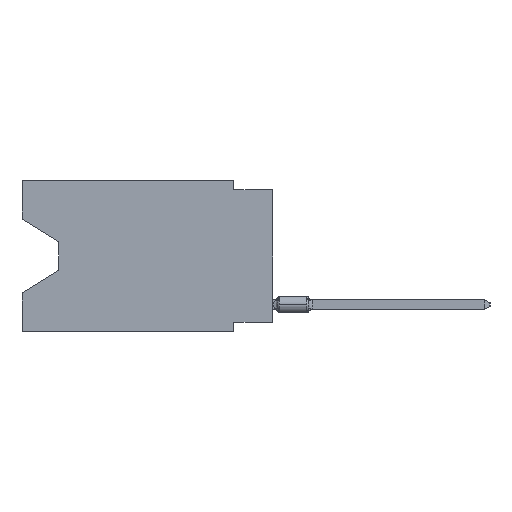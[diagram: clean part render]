
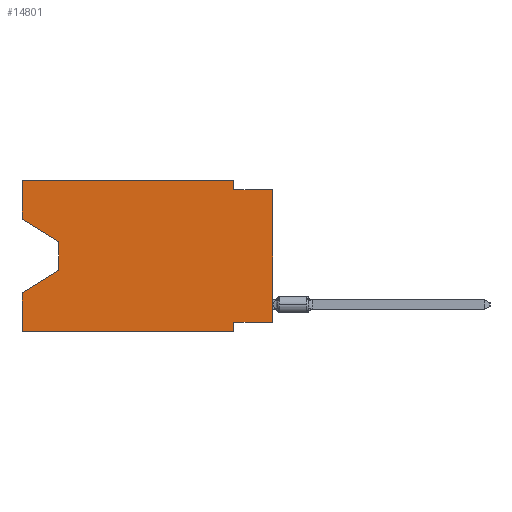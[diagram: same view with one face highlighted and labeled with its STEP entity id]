
A CAD part, left-side view. The second image highlights one B-rep face of the part: STEP entity #14801.
In plain terms, the highlighted planar face has unit normal (-1, 0, 0).
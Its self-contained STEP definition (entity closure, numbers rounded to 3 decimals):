
#1022 = EDGE_CURVE ( 'NONE', #17981, #5788, #20711, .T. ) ;
#1270 = VECTOR ( 'NONE', #9001, 1000. ) ;
#1369 = EDGE_CURVE ( 'NONE', #8016, #17981, #29683, .T. ) ;
#1737 = LINE ( 'NONE', #30207, #1270 ) ;
#1880 = VERTEX_POINT ( 'NONE', #11220 ) ;
#2065 = DIRECTION ( 'NONE',  ( 0., 0., -1. ) ) ;
#2238 = CARTESIAN_POINT ( 'NONE',  ( 0., 0., 0. ) ) ;
#2317 = CARTESIAN_POINT ( 'NONE',  ( 0., 0., -9.271 ) ) ;
#2870 = ORIENTED_EDGE ( 'NONE', *, *, #5244, .F. ) ;
#3889 = VERTEX_POINT ( 'NONE', #9206 ) ;
#4088 = VECTOR ( 'NONE', #12786, 1000. ) ;
#4113 = VECTOR ( 'NONE', #10424, 1000. ) ;
#4931 = LINE ( 'NONE', #23221, #11529 ) ;
#4990 = EDGE_CURVE ( 'NONE', #3889, #19101, #4931, .T. ) ;
#5244 = EDGE_CURVE ( 'NONE', #27262, #8016, #30579, .T. ) ;
#5245 = CARTESIAN_POINT ( 'NONE',  ( 0., 0., -0.635 ) ) ;
#5788 = VERTEX_POINT ( 'NONE', #13596 ) ;
#8016 = VERTEX_POINT ( 'NONE', #12560 ) ;
#8022 = CARTESIAN_POINT ( 'NONE',  ( 0., 16.383, 0. ) ) ;
#8332 = DIRECTION ( 'NONE',  ( 0., -1., 0. ) ) ;
#8886 = ORIENTED_EDGE ( 'NONE', *, *, #13821, .F. ) ;
#9001 = DIRECTION ( 'NONE',  ( 0., 0.855, -0.519 ) ) ;
#9114 = CARTESIAN_POINT ( 'NONE',  ( 0., 2.54, -9.906 ) ) ;
#9206 = CARTESIAN_POINT ( 'NONE',  ( 0., 13.97, -4.013 ) ) ;
#9372 = DIRECTION ( 'NONE',  ( 0., 0., 1. ) ) ;
#9789 = EDGE_CURVE ( 'NONE', #27262, #3889, #12582, .T. ) ;
#10093 = EDGE_CURVE ( 'NONE', #19101, #22108, #1737, .T. ) ;
#10105 = CARTESIAN_POINT ( 'NONE',  ( 0., 16.383, -2.546 ) ) ;
#10164 = LINE ( 'NONE', #24702, #4088 ) ;
#10324 = CARTESIAN_POINT ( 'NONE',  ( 0., 13.97, -5.893 ) ) ;
#10424 = DIRECTION ( 'NONE',  ( 0., 0., 1. ) ) ;
#10769 = VERTEX_POINT ( 'NONE', #9114 ) ;
#11010 = CARTESIAN_POINT ( 'NONE',  ( 0., 2.54, -9.271 ) ) ;
#11053 = FACE_OUTER_BOUND ( 'NONE', #19611, .T. ) ;
#11220 = CARTESIAN_POINT ( 'NONE',  ( 0., 0., -0.635 ) ) ;
#11428 = CARTESIAN_POINT ( 'NONE',  ( 0., 16.383, -9.906 ) ) ;
#11510 = ORIENTED_EDGE ( 'NONE', *, *, #22002, .T. ) ;
#11529 = VECTOR ( 'NONE', #14370, 1000. ) ;
#11697 = CARTESIAN_POINT ( 'NONE',  ( 0., 16.383, 0. ) ) ;
#12560 = CARTESIAN_POINT ( 'NONE',  ( 0., 16.383, 0. ) ) ;
#12582 = LINE ( 'NONE', #10105, #28963 ) ;
#12786 = DIRECTION ( 'NONE',  ( 0., 0., -1. ) ) ;
#13006 = ORIENTED_EDGE ( 'NONE', *, *, #17110, .F. ) ;
#13370 = PLANE ( 'NONE',  #16900 ) ;
#13426 = CARTESIAN_POINT ( 'NONE',  ( 0., 2.54, 0. ) ) ;
#13473 = VECTOR ( 'NONE', #23375, 1000. ) ;
#13487 = ORIENTED_EDGE ( 'NONE', *, *, #1369, .F. ) ;
#13596 = CARTESIAN_POINT ( 'NONE',  ( 0., 2.54, -0.635 ) ) ;
#13754 = CARTESIAN_POINT ( 'NONE',  ( 0., 16.383, -9.906 ) ) ;
#13759 = LINE ( 'NONE', #11428, #17284 ) ;
#13821 = EDGE_CURVE ( 'NONE', #24802, #10769, #10164, .T. ) ;
#14370 = DIRECTION ( 'NONE',  ( 0., 0., -1. ) ) ;
#14801 = ADVANCED_FACE ( 'NONE', ( #11053 ), #13370, .F. ) ;
#14821 = CARTESIAN_POINT ( 'NONE',  ( 0., 16.383, -7.36 ) ) ;
#14868 = VECTOR ( 'NONE', #30140, 1000. ) ;
#14977 = DIRECTION ( 'NONE',  ( 0., -1., 0. ) ) ;
#15236 = CARTESIAN_POINT ( 'NONE',  ( 0., 16.383, 0. ) ) ;
#15493 = VECTOR ( 'NONE', #9372, 1000. ) ;
#16236 = DIRECTION ( 'NONE',  ( 0., -1., 0. ) ) ;
#16244 = CARTESIAN_POINT ( 'NONE',  ( 0., 2.54, 0. ) ) ;
#16626 = DIRECTION ( 'NONE',  ( 0., 0., 1. ) ) ;
#16900 = AXIS2_PLACEMENT_3D ( 'NONE', #20345, #18012, #2065 ) ;
#17066 = VECTOR ( 'NONE', #16626, 1000. ) ;
#17110 = EDGE_CURVE ( 'NONE', #5788, #1880, #26584, .T. ) ;
#17284 = VECTOR ( 'NONE', #16236, 1000. ) ;
#17375 = ORIENTED_EDGE ( 'NONE', *, *, #4990, .T. ) ;
#17699 = LINE ( 'NONE', #15236, #4113 ) ;
#17981 = VERTEX_POINT ( 'NONE', #16244 ) ;
#18012 = DIRECTION ( 'NONE',  ( 1., 0., 0. ) ) ;
#18861 = ORIENTED_EDGE ( 'NONE', *, *, #10093, .T. ) ;
#19101 = VERTEX_POINT ( 'NONE', #10324 ) ;
#19524 = VECTOR ( 'NONE', #14977, 1000. ) ;
#19566 = DIRECTION ( 'NONE',  ( 0., -0.855, -0.519 ) ) ;
#19611 = EDGE_LOOP ( 'NONE', ( #29803, #17375, #18861, #23090, #11510, #8886, #23498, #21616, #13006, #20417, #13487, #2870 ) ) ;
#19881 = CARTESIAN_POINT ( 'NONE',  ( 0., 16.383, -2.546 ) ) ;
#20345 = CARTESIAN_POINT ( 'NONE',  ( 0., 16.383, 0. ) ) ;
#20417 = ORIENTED_EDGE ( 'NONE', *, *, #1022, .F. ) ;
#20711 = LINE ( 'NONE', #13426, #14868 ) ;
#21264 = LINE ( 'NONE', #2238, #17066 ) ;
#21616 = ORIENTED_EDGE ( 'NONE', *, *, #30544, .T. ) ;
#22002 = EDGE_CURVE ( 'NONE', #29576, #10769, #13759, .T. ) ;
#22108 = VERTEX_POINT ( 'NONE', #14821 ) ;
#22780 = VECTOR ( 'NONE', #8332, 1000. ) ;
#23090 = ORIENTED_EDGE ( 'NONE', *, *, #27341, .F. ) ;
#23221 = CARTESIAN_POINT ( 'NONE',  ( 0., 13.97, -4.013 ) ) ;
#23375 = DIRECTION ( 'NONE',  ( 0., 1., 0. ) ) ;
#23498 = ORIENTED_EDGE ( 'NONE', *, *, #26764, .F. ) ;
#24702 = CARTESIAN_POINT ( 'NONE',  ( 0., 2.54, -9.906 ) ) ;
#24802 = VERTEX_POINT ( 'NONE', #11010 ) ;
#26584 = LINE ( 'NONE', #5245, #19524 ) ;
#26764 = EDGE_CURVE ( 'NONE', #30163, #24802, #28324, .T. ) ;
#27262 = VERTEX_POINT ( 'NONE', #19881 ) ;
#27341 = EDGE_CURVE ( 'NONE', #29576, #22108, #17699, .T. ) ;
#28130 = CARTESIAN_POINT ( 'NONE',  ( 0., 0., -9.271 ) ) ;
#28324 = LINE ( 'NONE', #2317, #13473 ) ;
#28963 = VECTOR ( 'NONE', #19566, 1000. ) ;
#29576 = VERTEX_POINT ( 'NONE', #13754 ) ;
#29683 = LINE ( 'NONE', #8022, #22780 ) ;
#29803 = ORIENTED_EDGE ( 'NONE', *, *, #9789, .T. ) ;
#30140 = DIRECTION ( 'NONE',  ( 0., 0., -1. ) ) ;
#30163 = VERTEX_POINT ( 'NONE', #28130 ) ;
#30207 = CARTESIAN_POINT ( 'NONE',  ( 0., 13.97, -5.893 ) ) ;
#30544 = EDGE_CURVE ( 'NONE', #30163, #1880, #21264, .T. ) ;
#30579 = LINE ( 'NONE', #11697, #15493 ) ;
